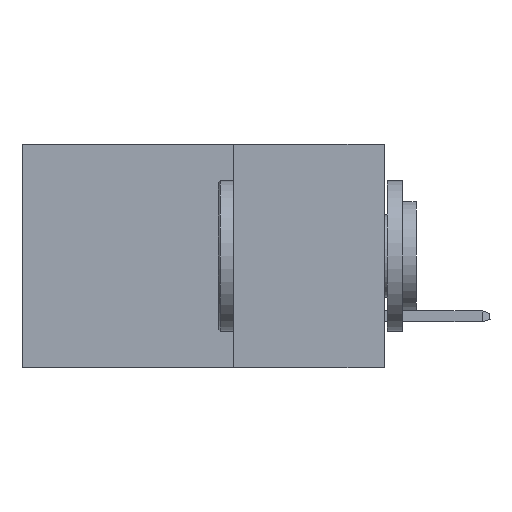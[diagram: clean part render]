
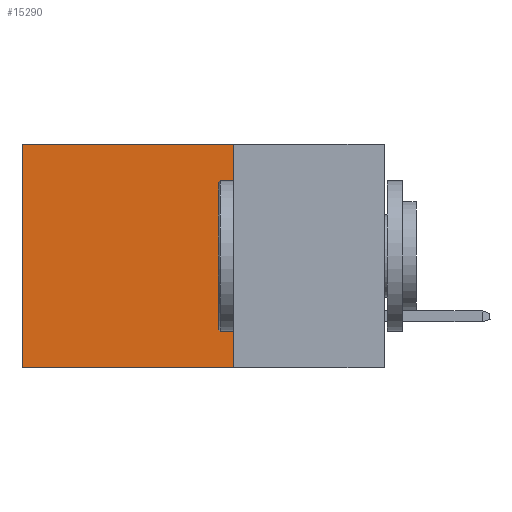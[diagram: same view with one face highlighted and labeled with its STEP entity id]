
A CAD part, left-side view. The second image highlights one B-rep face of the part: STEP entity #15290.
In plain terms, the highlighted planar face has unit normal (-1, 0, 0).
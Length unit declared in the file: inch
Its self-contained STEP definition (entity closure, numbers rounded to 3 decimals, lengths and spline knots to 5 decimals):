
#497 = DIRECTION ( 'NONE',  ( 0., 0., -1. ) ) ;
#712 = VECTOR ( 'NONE', #7755, 39.37008 ) ;
#1360 = CARTESIAN_POINT ( 'NONE',  ( 0.298, 0.25, 0. ) ) ;
#1920 = VERTEX_POINT ( 'NONE', #10361 ) ;
#2181 = ORIENTED_EDGE ( 'NONE', *, *, #12894, .T. ) ;
#2516 = LINE ( 'NONE', #16342, #9174 ) ;
#2540 = VERTEX_POINT ( 'NONE', #13293 ) ;
#2726 = CARTESIAN_POINT ( 'NONE',  ( 0.298, 0.25, 0. ) ) ;
#3203 = LINE ( 'NONE', #11748, #712 ) ;
#3350 = ORIENTED_EDGE ( 'NONE', *, *, #13704, .F. ) ;
#3717 = VECTOR ( 'NONE', #11960, 39.37008 ) ;
#4791 = VERTEX_POINT ( 'NONE', #8792 ) ;
#5103 = ORIENTED_EDGE ( 'NONE', *, *, #6515, .F. ) ;
#5517 = PLANE ( 'NONE',  #14856 ) ;
#5823 = EDGE_CURVE ( 'NONE', #2540, #8059, #2516, .T. ) ;
#6515 = EDGE_CURVE ( 'NONE', #1920, #4791, #12632, .T. ) ;
#6522 = LINE ( 'NONE', #8750, #10854 ) ;
#7755 = DIRECTION ( 'NONE',  ( 0., 1., 0. ) ) ;
#8049 = DIRECTION ( 'NONE',  ( 0., 0., -1. ) ) ;
#8059 = VERTEX_POINT ( 'NONE', #10625 ) ;
#8729 = FACE_OUTER_BOUND ( 'NONE', #17204, .T. ) ;
#8750 = CARTESIAN_POINT ( 'NONE',  ( 0.298, 0.25, -0.37 ) ) ;
#8792 = CARTESIAN_POINT ( 'NONE',  ( 0.298, 0.25, -0.37 ) ) ;
#9174 = VECTOR ( 'NONE', #497, 39.37008 ) ;
#10361 = CARTESIAN_POINT ( 'NONE',  ( 0.298, 0.25, 0. ) ) ;
#10625 = CARTESIAN_POINT ( 'NONE',  ( 0.298, 0.6, -0.37 ) ) ;
#10854 = VECTOR ( 'NONE', #11527, 39.37008 ) ;
#11527 = DIRECTION ( 'NONE',  ( 0., 1., 0. ) ) ;
#11748 = CARTESIAN_POINT ( 'NONE',  ( 0.298, 0.25, 0. ) ) ;
#11960 = DIRECTION ( 'NONE',  ( 0., 0., -1. ) ) ;
#12632 = LINE ( 'NONE', #1360, #3717 ) ;
#12894 = EDGE_CURVE ( 'NONE', #1920, #2540, #3203, .T. ) ;
#13293 = CARTESIAN_POINT ( 'NONE',  ( 0.298, 0.6, 0. ) ) ;
#13704 = EDGE_CURVE ( 'NONE', #4791, #8059, #6522, .T. ) ;
#14795 = DIRECTION ( 'NONE',  ( 1., 0., 0. ) ) ;
#14856 = AXIS2_PLACEMENT_3D ( 'NONE', #2726, #14795, #8049 ) ;
#15290 = ADVANCED_FACE ( 'NONE', ( #8729 ), #5517, .F. ) ;
#16018 = ORIENTED_EDGE ( 'NONE', *, *, #5823, .T. ) ;
#16342 = CARTESIAN_POINT ( 'NONE',  ( 0.298, 0.6, 0. ) ) ;
#17204 = EDGE_LOOP ( 'NONE', ( #16018, #3350, #5103, #2181 ) ) ;
